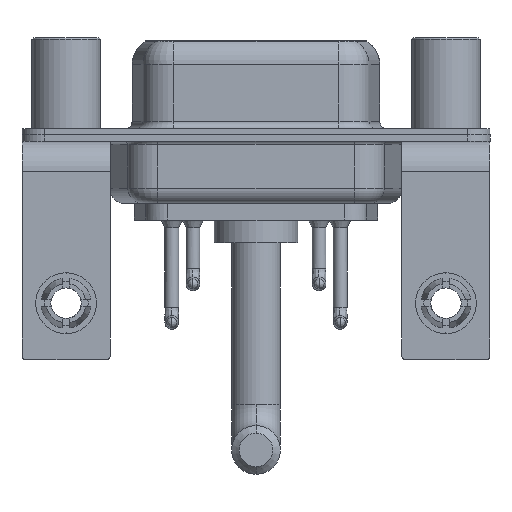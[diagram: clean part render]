
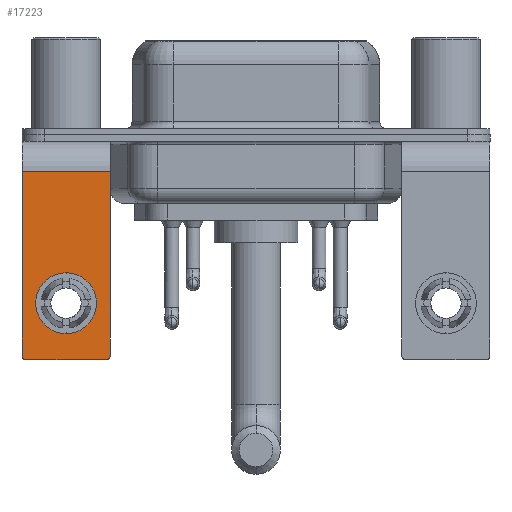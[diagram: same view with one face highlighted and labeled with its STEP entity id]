
A CAD part, front view. The second image highlights one B-rep face of the part: STEP entity #17223.
In plain terms, the highlighted planar face has unit normal (0, -1, 0).
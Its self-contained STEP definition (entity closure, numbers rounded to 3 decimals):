
#279 = EDGE_CURVE ( 'NONE', #6179, #14381, #929, .T. ) ;
#311 = CARTESIAN_POINT ( 'NONE',  ( -2.9, -6.25, -2.4 ) ) ;
#389 = CARTESIAN_POINT ( 'NONE',  ( 0., -6.25, -13.07 ) ) ;
#820 = EDGE_LOOP ( 'NONE', ( #13329, #4164, #2525, #19003, #10728, #11951 ) ) ;
#929 = CIRCLE ( 'NONE', #8514, 0.25 ) ;
#1002 = AXIS2_PLACEMENT_3D ( 'NONE', #3825, #6912, #14777 ) ;
#1100 = CARTESIAN_POINT ( 'NONE',  ( 2.9, -6.25, -2.4 ) ) ;
#1215 = CARTESIAN_POINT ( 'NONE',  ( 2.65, -6.25, -14.55 ) ) ;
#1758 = VECTOR ( 'NONE', #4279, 1000. ) ;
#2525 = ORIENTED_EDGE ( 'NONE', *, *, #18691, .F. ) ;
#2876 = ORIENTED_EDGE ( 'NONE', *, *, #12202, .T. ) ;
#3825 = CARTESIAN_POINT ( 'NONE',  ( 0., -6.25, -11.07 ) ) ;
#4042 = EDGE_CURVE ( 'NONE', #12436, #14381, #13161, .T. ) ;
#4163 = DIRECTION ( 'NONE',  ( 0., 0., 1. ) ) ;
#4164 = ORIENTED_EDGE ( 'NONE', *, *, #12702, .T. ) ;
#4258 = DIRECTION ( 'NONE',  ( 0., -1., 0. ) ) ;
#4279 = DIRECTION ( 'NONE',  ( -1., 0., 0. ) ) ;
#5423 = CARTESIAN_POINT ( 'NONE',  ( 2.9, -6.25, -2.4 ) ) ;
#5426 = CARTESIAN_POINT ( 'NONE',  ( 2.9, -6.25, -14.8 ) ) ;
#5920 = CIRCLE ( 'NONE', #1002, 2. ) ;
#6179 = VERTEX_POINT ( 'NONE', #16568 ) ;
#6912 = DIRECTION ( 'NONE',  ( 0., 1., 0. ) ) ;
#6972 = LINE ( 'NONE', #5426, #10023 ) ;
#7160 = EDGE_CURVE ( 'NONE', #12436, #7236, #7491, .T. ) ;
#7218 = VECTOR ( 'NONE', #8041, 1000. ) ;
#7236 = VERTEX_POINT ( 'NONE', #12557 ) ;
#7360 = VERTEX_POINT ( 'NONE', #14517 ) ;
#7491 = LINE ( 'NONE', #1100, #1758 ) ;
#7981 = AXIS2_PLACEMENT_3D ( 'NONE', #5423, #13577, #19518 ) ;
#8041 = DIRECTION ( 'NONE',  ( 0., 0., -1. ) ) ;
#8514 = AXIS2_PLACEMENT_3D ( 'NONE', #1215, #12154, #10303 ) ;
#8580 = VERTEX_POINT ( 'NONE', #11486 ) ;
#8661 = AXIS2_PLACEMENT_3D ( 'NONE', #10676, #17002, #12039 ) ;
#8837 = FACE_BOUND ( 'NONE', #14727, .T. ) ;
#9324 = VERTEX_POINT ( 'NONE', #389 ) ;
#9357 = CARTESIAN_POINT ( 'NONE',  ( -2.65, -6.25, -14.8 ) ) ;
#9790 = ORIENTED_EDGE ( 'NONE', *, *, #14929, .T. ) ;
#10023 = VECTOR ( 'NONE', #11713, 1000. ) ;
#10303 = DIRECTION ( 'NONE',  ( 0., 0., 1. ) ) ;
#10676 = CARTESIAN_POINT ( 'NONE',  ( 0., -6.25, -11.07 ) ) ;
#10728 = ORIENTED_EDGE ( 'NONE', *, *, #4042, .F. ) ;
#11486 = CARTESIAN_POINT ( 'NONE',  ( 0., -6.25, -9.07 ) ) ;
#11713 = DIRECTION ( 'NONE',  ( -1., 0., 0. ) ) ;
#11951 = ORIENTED_EDGE ( 'NONE', *, *, #7160, .T. ) ;
#12039 = DIRECTION ( 'NONE',  ( 0., 0., 1. ) ) ;
#12154 = DIRECTION ( 'NONE',  ( 0., -1., 0. ) ) ;
#12202 = EDGE_CURVE ( 'NONE', #9324, #8580, #16895, .T. ) ;
#12436 = VERTEX_POINT ( 'NONE', #14213 ) ;
#12557 = CARTESIAN_POINT ( 'NONE',  ( -2.9, -6.25, -2.4 ) ) ;
#12702 = EDGE_CURVE ( 'NONE', #7360, #17011, #19433, .T. ) ;
#13161 = LINE ( 'NONE', #18027, #17339 ) ;
#13329 = ORIENTED_EDGE ( 'NONE', *, *, #13384, .T. ) ;
#13384 = EDGE_CURVE ( 'NONE', #7236, #7360, #19009, .T. ) ;
#13491 = PLANE ( 'NONE',  #7981 ) ;
#13577 = DIRECTION ( 'NONE',  ( 0., 1., 0. ) ) ;
#14213 = CARTESIAN_POINT ( 'NONE',  ( 2.9, -6.25, -2.4 ) ) ;
#14381 = VERTEX_POINT ( 'NONE', #14590 ) ;
#14415 = DIRECTION ( 'NONE',  ( 0., 0., -1. ) ) ;
#14517 = CARTESIAN_POINT ( 'NONE',  ( -2.9, -6.25, -14.55 ) ) ;
#14590 = CARTESIAN_POINT ( 'NONE',  ( 2.9, -6.25, -14.55 ) ) ;
#14727 = EDGE_LOOP ( 'NONE', ( #2876, #9790 ) ) ;
#14777 = DIRECTION ( 'NONE',  ( 0., 0., 1. ) ) ;
#14929 = EDGE_CURVE ( 'NONE', #8580, #9324, #5920, .T. ) ;
#15443 = AXIS2_PLACEMENT_3D ( 'NONE', #18335, #4258, #4163 ) ;
#16568 = CARTESIAN_POINT ( 'NONE',  ( 2.65, -6.25, -14.8 ) ) ;
#16895 = CIRCLE ( 'NONE', #8661, 2. ) ;
#17002 = DIRECTION ( 'NONE',  ( 0., 1., 0. ) ) ;
#17011 = VERTEX_POINT ( 'NONE', #9357 ) ;
#17223 = ADVANCED_FACE ( 'NONE', ( #8837, #19620 ), #13491, .F. ) ;
#17339 = VECTOR ( 'NONE', #14415, 1000. ) ;
#18027 = CARTESIAN_POINT ( 'NONE',  ( 2.9, -6.25, -2.4 ) ) ;
#18335 = CARTESIAN_POINT ( 'NONE',  ( -2.65, -6.25, -14.55 ) ) ;
#18691 = EDGE_CURVE ( 'NONE', #6179, #17011, #6972, .T. ) ;
#19003 = ORIENTED_EDGE ( 'NONE', *, *, #279, .T. ) ;
#19009 = LINE ( 'NONE', #311, #7218 ) ;
#19433 = CIRCLE ( 'NONE', #15443, 0.25 ) ;
#19518 = DIRECTION ( 'NONE',  ( 0., 0., 1. ) ) ;
#19620 = FACE_OUTER_BOUND ( 'NONE', #820, .T. ) ;
